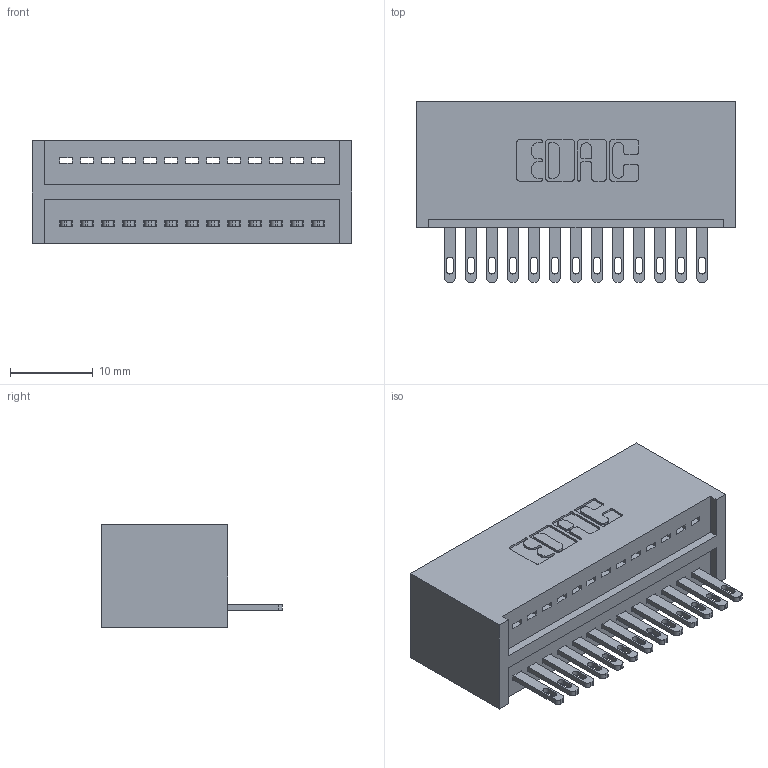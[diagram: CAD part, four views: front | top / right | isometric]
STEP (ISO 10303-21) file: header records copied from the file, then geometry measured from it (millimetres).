
FILE_DESCRIPTION (( 'STEP AP203' ), '1' );
FILE_NAME ('325-013-500-101.STEP', '2020-02-24T15:37:46', ( '' ), ( '' ), 'SwSTEP 2.0', 'SolidWorks 2016', '' );
FILE_SCHEMA (( 'CONFIG_CONTROL_DESIGN' ));
Length unit declared in the file: inch
Products named in the file (3): 325-013-500-101; 325-292-001_325-293-100; 325 Part_Lugless
Assembly tree (14 placements, depth 2):
  325-013-500-101
    325 Part_Lugless
    325-292-001_325-293-100  x13
Bounding box: 38.66 x 21.84 x 12.45 mm (x, y, z)
Volume: 5259.4 mm3; surface area: 5774.8 mm2
Topology: 14 solids, 14 shells, 808 faces, 2471 edges, 1646 vertices
Faces by surface type: plane 534, cylinder 274
Entity records: 11351 total; most frequent: CARTESIAN_POINT 1969, ORIENTED_EDGE 1918, DIRECTION 1713, EDGE_CURVE 959, LINE 835, VECTOR 835, VERTEX_POINT 638, AXIS2_PLACEMENT_3D 439
